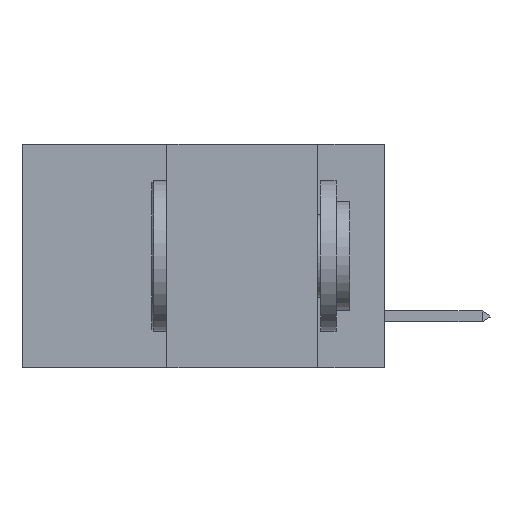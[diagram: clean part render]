
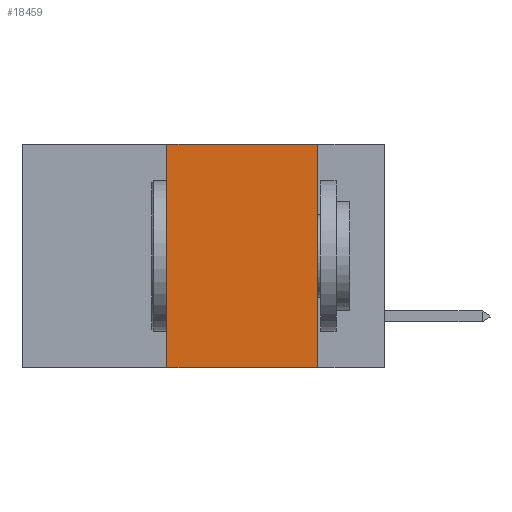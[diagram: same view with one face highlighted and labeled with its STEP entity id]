
A CAD part, left-side view. The second image highlights one B-rep face of the part: STEP entity #18459.
In plain terms, the highlighted planar face has unit normal (-1, 0, 0).
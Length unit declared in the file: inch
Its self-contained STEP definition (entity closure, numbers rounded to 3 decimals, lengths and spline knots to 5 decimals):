
#230 = CARTESIAN_POINT ( 'NONE',  ( 0., 0.11, -0.37 ) ) ;
#589 = CARTESIAN_POINT ( 'NONE',  ( 0., 0.6, 0. ) ) ;
#1327 = VERTEX_POINT ( 'NONE', #14488 ) ;
#1631 = EDGE_CURVE ( 'NONE', #18303, #10670, #8431, .T. ) ;
#1950 = ORIENTED_EDGE ( 'NONE', *, *, #1631, .F. ) ;
#2059 = DIRECTION ( 'NONE',  ( 1., 0., 0. ) ) ;
#3674 = DIRECTION ( 'NONE',  ( 0., 0., -1. ) ) ;
#3910 = VERTEX_POINT ( 'NONE', #8332 ) ;
#4851 = DIRECTION ( 'NONE',  ( 0., 0., 1. ) ) ;
#4920 = CARTESIAN_POINT ( 'NONE',  ( 0., 0.36, 0. ) ) ;
#5463 = VECTOR ( 'NONE', #4851, 39.37008 ) ;
#5744 = DIRECTION ( 'NONE',  ( 0., -1., 0. ) ) ;
#6202 = EDGE_CURVE ( 'NONE', #3910, #10670, #11513, .T. ) ;
#6366 = ORIENTED_EDGE ( 'NONE', *, *, #19896, .F. ) ;
#7672 = EDGE_LOOP ( 'NONE', ( #1950, #6366, #15813, #13850 ) ) ;
#8332 = CARTESIAN_POINT ( 'NONE',  ( 0., 0.36, -0.37 ) ) ;
#8431 = LINE ( 'NONE', #20744, #13199 ) ;
#9455 = DIRECTION ( 'NONE',  ( 0., -1., 0. ) ) ;
#10220 = CARTESIAN_POINT ( 'NONE',  ( 0., 0.6, -0.37 ) ) ;
#10670 = VERTEX_POINT ( 'NONE', #230 ) ;
#11513 = LINE ( 'NONE', #10220, #19303 ) ;
#12381 = CARTESIAN_POINT ( 'NONE',  ( 0., 0.6, 0. ) ) ;
#12434 = VECTOR ( 'NONE', #9455, 39.37008 ) ;
#13199 = VECTOR ( 'NONE', #17702, 39.37008 ) ;
#13850 = ORIENTED_EDGE ( 'NONE', *, *, #6202, .T. ) ;
#14488 = CARTESIAN_POINT ( 'NONE',  ( 0., 0.36, 0. ) ) ;
#14693 = CARTESIAN_POINT ( 'NONE',  ( 0., 0.11, 0. ) ) ;
#14757 = LINE ( 'NONE', #4920, #5463 ) ;
#15463 = LINE ( 'NONE', #12381, #12434 ) ;
#15813 = ORIENTED_EDGE ( 'NONE', *, *, #18920, .F. ) ;
#17046 = FACE_OUTER_BOUND ( 'NONE', #7672, .T. ) ;
#17702 = DIRECTION ( 'NONE',  ( 0., 0., -1. ) ) ;
#18303 = VERTEX_POINT ( 'NONE', #14693 ) ;
#18459 = ADVANCED_FACE ( 'NONE', ( #17046 ), #19820, .F. ) ;
#18920 = EDGE_CURVE ( 'NONE', #3910, #1327, #14757, .T. ) ;
#19303 = VECTOR ( 'NONE', #5744, 39.37008 ) ;
#19820 = PLANE ( 'NONE',  #19920 ) ;
#19896 = EDGE_CURVE ( 'NONE', #1327, #18303, #15463, .T. ) ;
#19920 = AXIS2_PLACEMENT_3D ( 'NONE', #589, #2059, #3674 ) ;
#20744 = CARTESIAN_POINT ( 'NONE',  ( 0., 0.11, 0. ) ) ;
